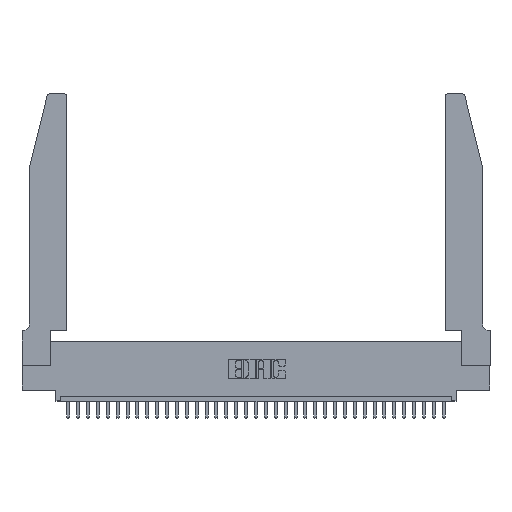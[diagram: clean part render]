
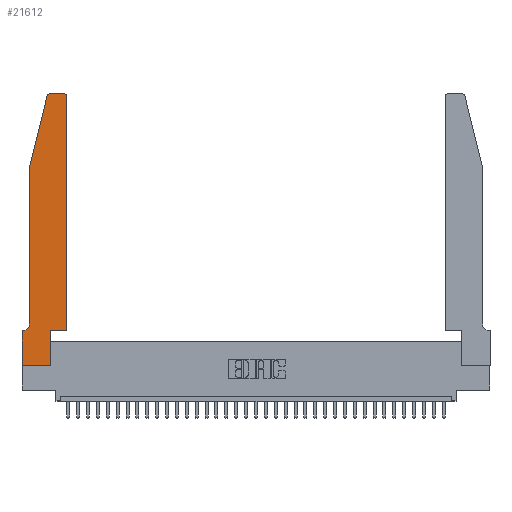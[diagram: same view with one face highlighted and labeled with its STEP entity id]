
A CAD part, top view. The second image highlights one B-rep face of the part: STEP entity #21612.
In plain terms, the highlighted planar face has unit normal (0, 0, 1).
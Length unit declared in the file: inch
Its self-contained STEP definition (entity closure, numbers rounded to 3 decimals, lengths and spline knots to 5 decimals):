
#239 = CARTESIAN_POINT ( 'NONE',  ( 0.0055, 0.42, 0.37 ) ) ;
#459 = DIRECTION ( 'NONE',  ( -1., 0., 0. ) ) ;
#969 = DIRECTION ( 'NONE',  ( 0., -1., 0. ) ) ;
#2062 = VERTEX_POINT ( 'NONE', #2530 ) ;
#2275 = ORIENTED_EDGE ( 'NONE', *, *, #21639, .T. ) ;
#2310 = DIRECTION ( 'NONE',  ( 0., 0., 1. ) ) ;
#2477 = EDGE_CURVE ( 'NONE', #2062, #11034, #18430, .T. ) ;
#2530 = CARTESIAN_POINT ( 'NONE',  ( 0.25487, 2.72718, 0.37 ) ) ;
#2712 = ORIENTED_EDGE ( 'NONE', *, *, #28683, .T. ) ;
#3037 = CIRCLE ( 'NONE', #11553, 0.07 ) ;
#3075 = EDGE_LOOP ( 'NONE', ( #13531, #12920, #9775, #28938, #10157, #11345, #31475, #2712, #5897, #29735, #2275, #23228 ) ) ;
#3286 = VECTOR ( 'NONE', #30665, 39.37008 ) ;
#3645 = EDGE_CURVE ( 'NONE', #6419, #2062, #18745, .T. ) ;
#3708 = VERTEX_POINT ( 'NONE', #16458 ) ;
#4303 = CARTESIAN_POINT ( 'NONE',  ( 0.0055, 0.35, 0.37 ) ) ;
#4351 = DIRECTION ( 'NONE',  ( 1., 0., 0. ) ) ;
#4639 = VERTEX_POINT ( 'NONE', #17641 ) ;
#5308 = VERTEX_POINT ( 'NONE', #29315 ) ;
#5446 = CARTESIAN_POINT ( 'NONE',  ( 0.2865, 0.35, 0.37 ) ) ;
#5685 = DIRECTION ( 'NONE',  ( -1., 0., 0. ) ) ;
#5859 = VECTOR ( 'NONE', #11559, 39.37008 ) ;
#5897 = ORIENTED_EDGE ( 'NONE', *, *, #5929, .T. ) ;
#5908 = LINE ( 'NONE', #7073, #7234 ) ;
#5929 = EDGE_CURVE ( 'NONE', #15501, #15373, #8162, .T. ) ;
#6419 = VERTEX_POINT ( 'NONE', #34389 ) ;
#6827 = VECTOR ( 'NONE', #13966, 39.37008 ) ;
#7073 = CARTESIAN_POINT ( 'NONE',  ( 0.4505, 0.35, 0.37 ) ) ;
#7234 = VECTOR ( 'NONE', #4351, 39.37008 ) ;
#8162 = LINE ( 'NONE', #5446, #13575 ) ;
#8607 = PLANE ( 'NONE',  #23886 ) ;
#9222 = LINE ( 'NONE', #34182, #21734 ) ;
#9775 = ORIENTED_EDGE ( 'NONE', *, *, #2477, .T. ) ;
#9918 = VECTOR ( 'NONE', #969, 39.37008 ) ;
#10157 = ORIENTED_EDGE ( 'NONE', *, *, #31913, .T. ) ;
#10342 = CARTESIAN_POINT ( 'NONE',  ( 0.284, 2.72, 0.37 ) ) ;
#11034 = VERTEX_POINT ( 'NONE', #19786 ) ;
#11345 = ORIENTED_EDGE ( 'NONE', *, *, #24893, .T. ) ;
#11553 = AXIS2_PLACEMENT_3D ( 'NONE', #239, #13574, #5685 ) ;
#11559 = DIRECTION ( 'NONE',  ( 0., 1., 0. ) ) ;
#12219 = DIRECTION ( 'NONE',  ( 0., 0., 1. ) ) ;
#12224 = FACE_OUTER_BOUND ( 'NONE', #3075, .T. ) ;
#12920 = ORIENTED_EDGE ( 'NONE', *, *, #3645, .T. ) ;
#13063 = LINE ( 'NONE', #16766, #5859 ) ;
#13531 = ORIENTED_EDGE ( 'NONE', *, *, #19649, .T. ) ;
#13574 = DIRECTION ( 'NONE',  ( 0., 0., -1. ) ) ;
#13575 = VECTOR ( 'NONE', #24155, 39.37008 ) ;
#13966 = DIRECTION ( 'NONE',  ( 0., -1., 0. ) ) ;
#13997 = CARTESIAN_POINT ( 'NONE',  ( 0., 0., 0.37 ) ) ;
#14063 = LINE ( 'NONE', #21801, #17413 ) ;
#14091 = CARTESIAN_POINT ( 'NONE',  ( 0.2865, 0., 0.37 ) ) ;
#15010 = VERTEX_POINT ( 'NONE', #4303 ) ;
#15373 = VERTEX_POINT ( 'NONE', #32755 ) ;
#15501 = VERTEX_POINT ( 'NONE', #14091 ) ;
#16458 = CARTESIAN_POINT ( 'NONE',  ( 0.4205, 2.75, 0.37 ) ) ;
#16670 = VERTEX_POINT ( 'NONE', #32563 ) ;
#16766 = CARTESIAN_POINT ( 'NONE',  ( 0.4505, 0.35, 0.37 ) ) ;
#17413 = VECTOR ( 'NONE', #459, 39.37008 ) ;
#17547 = CARTESIAN_POINT ( 'NONE',  ( 0.4205, 2.72, 0.37 ) ) ;
#17641 = CARTESIAN_POINT ( 'NONE',  ( 0.0755, 0.42, 0.37 ) ) ;
#18430 = LINE ( 'NONE', #22781, #3286 ) ;
#18745 = CIRCLE ( 'NONE', #21530, 0.03 ) ;
#18781 = VERTEX_POINT ( 'NONE', #30481 ) ;
#19649 = EDGE_CURVE ( 'NONE', #3708, #6419, #31601, .T. ) ;
#19786 = CARTESIAN_POINT ( 'NONE',  ( 0.0755, 2., 0.37 ) ) ;
#19895 = DIRECTION ( 'NONE',  ( 1., 0., 0. ) ) ;
#20598 = EDGE_CURVE ( 'NONE', #11034, #4639, #32776, .T. ) ;
#20720 = CIRCLE ( 'NONE', #21196, 0.03 ) ;
#21196 = AXIS2_PLACEMENT_3D ( 'NONE', #17547, #12219, #19895 ) ;
#21530 = AXIS2_PLACEMENT_3D ( 'NONE', #10342, #2310, #25001 ) ;
#21612 = ADVANCED_FACE ( 'NONE', ( #12224 ), #8607, .T. ) ;
#21639 = EDGE_CURVE ( 'NONE', #16670, #5308, #13063, .T. ) ;
#21734 = VECTOR ( 'NONE', #31382, 39.37008 ) ;
#21801 = CARTESIAN_POINT ( 'NONE',  ( 0.0755, 0.35, 0.37 ) ) ;
#22781 = CARTESIAN_POINT ( 'NONE',  ( 0.0755, 2., 0.37 ) ) ;
#22832 = CARTESIAN_POINT ( 'NONE',  ( 0.2605, 2.75, 0.37 ) ) ;
#23228 = ORIENTED_EDGE ( 'NONE', *, *, #31563, .T. ) ;
#23886 = AXIS2_PLACEMENT_3D ( 'NONE', #30288, #32877, #27338 ) ;
#24155 = DIRECTION ( 'NONE',  ( 0., 1., 0. ) ) ;
#24893 = EDGE_CURVE ( 'NONE', #15010, #18781, #14063, .T. ) ;
#25001 = DIRECTION ( 'NONE',  ( 1., 0., 0. ) ) ;
#25376 = LINE ( 'NONE', #13997, #9918 ) ;
#25556 = DIRECTION ( 'NONE',  ( -1., 0., 0. ) ) ;
#27274 = VECTOR ( 'NONE', #25556, 39.37008 ) ;
#27338 = DIRECTION ( 'NONE',  ( 1., 0., 0. ) ) ;
#27445 = EDGE_CURVE ( 'NONE', #15373, #16670, #5908, .T. ) ;
#28199 = CARTESIAN_POINT ( 'NONE',  ( 0., 0., 0.37 ) ) ;
#28617 = CARTESIAN_POINT ( 'NONE',  ( 0.0755, 2., 0.37 ) ) ;
#28683 = EDGE_CURVE ( 'NONE', #32126, #15501, #9222, .T. ) ;
#28938 = ORIENTED_EDGE ( 'NONE', *, *, #20598, .T. ) ;
#29315 = CARTESIAN_POINT ( 'NONE',  ( 0.4505, 2.72, 0.37 ) ) ;
#29735 = ORIENTED_EDGE ( 'NONE', *, *, #27445, .T. ) ;
#30288 = CARTESIAN_POINT ( 'NONE',  ( 0., 0.35, 0.37 ) ) ;
#30481 = CARTESIAN_POINT ( 'NONE',  ( 0., 0.35, 0.37 ) ) ;
#30665 = DIRECTION ( 'NONE',  ( -0.239, -0.971, 0. ) ) ;
#31382 = DIRECTION ( 'NONE',  ( 1., 0., 0. ) ) ;
#31475 = ORIENTED_EDGE ( 'NONE', *, *, #34562, .T. ) ;
#31563 = EDGE_CURVE ( 'NONE', #5308, #3708, #20720, .T. ) ;
#31601 = LINE ( 'NONE', #22832, #27274 ) ;
#31913 = EDGE_CURVE ( 'NONE', #4639, #15010, #3037, .T. ) ;
#32126 = VERTEX_POINT ( 'NONE', #28199 ) ;
#32563 = CARTESIAN_POINT ( 'NONE',  ( 0.4505, 0.35, 0.37 ) ) ;
#32755 = CARTESIAN_POINT ( 'NONE',  ( 0.2865, 0.35, 0.37 ) ) ;
#32776 = LINE ( 'NONE', #28617, #6827 ) ;
#32877 = DIRECTION ( 'NONE',  ( 0., 0., 1. ) ) ;
#34182 = CARTESIAN_POINT ( 'NONE',  ( 0., 0., 0.37 ) ) ;
#34389 = CARTESIAN_POINT ( 'NONE',  ( 0.284, 2.75, 0.37 ) ) ;
#34562 = EDGE_CURVE ( 'NONE', #18781, #32126, #25376, .T. ) ;
